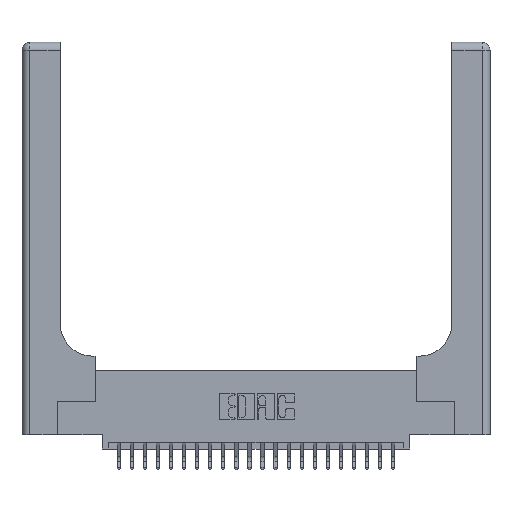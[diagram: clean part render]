
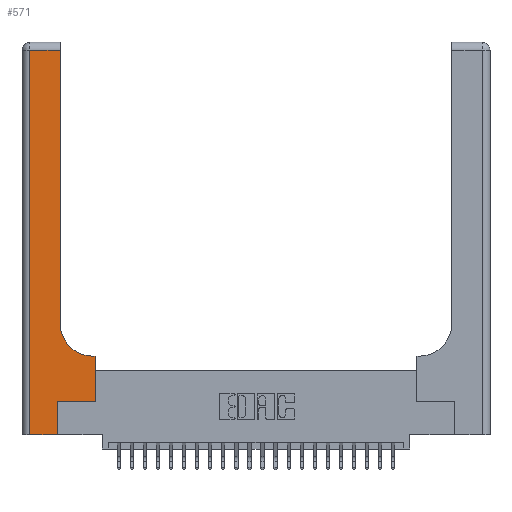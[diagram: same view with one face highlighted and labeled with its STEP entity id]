
A CAD part, top view. The second image highlights one B-rep face of the part: STEP entity #571.
In plain terms, the highlighted planar face has unit normal (0, 0, 1).
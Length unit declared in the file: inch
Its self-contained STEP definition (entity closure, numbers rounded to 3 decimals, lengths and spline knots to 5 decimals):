
#497 = FACE_OUTER_BOUND ( 'NONE', #19623, .T. ) ;
#571 = ADVANCED_FACE ( 'NONE', ( #497 ), #5939, .F. ) ;
#609 = VECTOR ( 'NONE', #12725, 39.37008 ) ;
#621 = ORIENTED_EDGE ( 'NONE', *, *, #16434, .T. ) ;
#748 = EDGE_CURVE ( 'NONE', #19835, #6950, #21726, .T. ) ;
#992 = LINE ( 'NONE', #1915, #19444 ) ;
#1112 = CARTESIAN_POINT ( 'NONE',  ( 0.269, 0., 0.37 ) ) ;
#1280 = VERTEX_POINT ( 'NONE', #1945 ) ;
#1745 = DIRECTION ( 'NONE',  ( -1., 0., 0. ) ) ;
#1761 = VECTOR ( 'NONE', #2232, 39.37008 ) ;
#1915 = CARTESIAN_POINT ( 'NONE',  ( 0., 2.94, 0.37 ) ) ;
#1945 = CARTESIAN_POINT ( 'NONE',  ( 0.5585, 0.25, 0.37 ) ) ;
#2232 = DIRECTION ( 'NONE',  ( 0., -1., 0. ) ) ;
#2864 = EDGE_CURVE ( 'NONE', #5690, #19835, #11714, .T. ) ;
#3074 = ORIENTED_EDGE ( 'NONE', *, *, #3219, .T. ) ;
#3219 = EDGE_CURVE ( 'NONE', #1280, #5690, #13541, .T. ) ;
#3828 = EDGE_CURVE ( 'NONE', #12616, #21300, #10769, .T. ) ;
#4509 = VERTEX_POINT ( 'NONE', #17120 ) ;
#4529 = LINE ( 'NONE', #17593, #23358 ) ;
#4808 = EDGE_CURVE ( 'NONE', #6348, #1280, #4529, .T. ) ;
#4870 = CARTESIAN_POINT ( 'NONE',  ( 0.5415, 0.85, 0.37 ) ) ;
#5559 = VECTOR ( 'NONE', #12147, 39.37008 ) ;
#5690 = VERTEX_POINT ( 'NONE', #9542 ) ;
#5762 = DIRECTION ( 'NONE',  ( 0., 0., -1. ) ) ;
#5939 = PLANE ( 'NONE',  #9701 ) ;
#6063 = EDGE_CURVE ( 'NONE', #4509, #12616, #10995, .T. ) ;
#6348 = VERTEX_POINT ( 'NONE', #20475 ) ;
#6451 = LINE ( 'NONE', #18669, #8583 ) ;
#6756 = VERTEX_POINT ( 'NONE', #10622 ) ;
#6950 = VERTEX_POINT ( 'NONE', #10412 ) ;
#7523 = CARTESIAN_POINT ( 'NONE',  ( 0.5415, 0.6, 0.37 ) ) ;
#7653 = ORIENTED_EDGE ( 'NONE', *, *, #24988, .T. ) ;
#8583 = VECTOR ( 'NONE', #21330, 39.37008 ) ;
#9542 = CARTESIAN_POINT ( 'NONE',  ( 0.5585, 0.6, 0.37 ) ) ;
#9701 = AXIS2_PLACEMENT_3D ( 'NONE', #15569, #5762, #9858 ) ;
#9739 = CARTESIAN_POINT ( 'NONE',  ( 0.06, 3., 0.37 ) ) ;
#9858 = DIRECTION ( 'NONE',  ( -1., 0., 0. ) ) ;
#10412 = CARTESIAN_POINT ( 'NONE',  ( 0.2915, 0.85, 0.37 ) ) ;
#10622 = CARTESIAN_POINT ( 'NONE',  ( 0.2915, 2.94, 0.37 ) ) ;
#10687 = CARTESIAN_POINT ( 'NONE',  ( 0.5585, 0.25, 0.37 ) ) ;
#10769 = LINE ( 'NONE', #21875, #5559 ) ;
#10995 = LINE ( 'NONE', #9739, #1761 ) ;
#11714 = LINE ( 'NONE', #15546, #15106 ) ;
#12147 = DIRECTION ( 'NONE',  ( 1., 0., 0. ) ) ;
#12616 = VERTEX_POINT ( 'NONE', #15488 ) ;
#12670 = DIRECTION ( 'NONE',  ( 1., 0., 0. ) ) ;
#12725 = DIRECTION ( 'NONE',  ( 0., 1., 0. ) ) ;
#13047 = EDGE_CURVE ( 'NONE', #21300, #6348, #24643, .T. ) ;
#13541 = LINE ( 'NONE', #10687, #609 ) ;
#15106 = VECTOR ( 'NONE', #15370, 39.37008 ) ;
#15365 = CARTESIAN_POINT ( 'NONE',  ( 0.269, 0., 0.37 ) ) ;
#15370 = DIRECTION ( 'NONE',  ( -1., 0., 0. ) ) ;
#15488 = CARTESIAN_POINT ( 'NONE',  ( 0.06, 0., 0.37 ) ) ;
#15546 = CARTESIAN_POINT ( 'NONE',  ( 0.2915, 0.6, 0.37 ) ) ;
#15569 = CARTESIAN_POINT ( 'NONE',  ( 0., 3., 0.37 ) ) ;
#16434 = EDGE_CURVE ( 'NONE', #6756, #4509, #992, .T. ) ;
#16769 = ORIENTED_EDGE ( 'NONE', *, *, #13047, .T. ) ;
#17120 = CARTESIAN_POINT ( 'NONE',  ( 0.06, 2.94, 0.37 ) ) ;
#17593 = CARTESIAN_POINT ( 'NONE',  ( 0.269, 0.25, 0.37 ) ) ;
#18669 = CARTESIAN_POINT ( 'NONE',  ( 0.2915, 3., 0.37 ) ) ;
#19250 = ORIENTED_EDGE ( 'NONE', *, *, #3828, .T. ) ;
#19358 = VECTOR ( 'NONE', #25365, 39.37008 ) ;
#19444 = VECTOR ( 'NONE', #1745, 39.37008 ) ;
#19623 = EDGE_LOOP ( 'NONE', ( #7653, #621, #21655, #19250, #16769, #24435, #3074, #21326, #19743 ) ) ;
#19743 = ORIENTED_EDGE ( 'NONE', *, *, #748, .T. ) ;
#19835 = VERTEX_POINT ( 'NONE', #7523 ) ;
#20215 = AXIS2_PLACEMENT_3D ( 'NONE', #4870, #22315, #12670 ) ;
#20475 = CARTESIAN_POINT ( 'NONE',  ( 0.269, 0.25, 0.37 ) ) ;
#21300 = VERTEX_POINT ( 'NONE', #1112 ) ;
#21326 = ORIENTED_EDGE ( 'NONE', *, *, #2864, .T. ) ;
#21330 = DIRECTION ( 'NONE',  ( 0., 1., 0. ) ) ;
#21655 = ORIENTED_EDGE ( 'NONE', *, *, #6063, .T. ) ;
#21726 = CIRCLE ( 'NONE', #20215, 0.25 ) ;
#21875 = CARTESIAN_POINT ( 'NONE',  ( 0., 0., 0.37 ) ) ;
#22315 = DIRECTION ( 'NONE',  ( 0., 0., -1. ) ) ;
#23358 = VECTOR ( 'NONE', #23568, 39.37008 ) ;
#23568 = DIRECTION ( 'NONE',  ( 1., 0., 0. ) ) ;
#24435 = ORIENTED_EDGE ( 'NONE', *, *, #4808, .T. ) ;
#24643 = LINE ( 'NONE', #15365, #19358 ) ;
#24988 = EDGE_CURVE ( 'NONE', #6950, #6756, #6451, .T. ) ;
#25365 = DIRECTION ( 'NONE',  ( 0., 1., 0. ) ) ;
